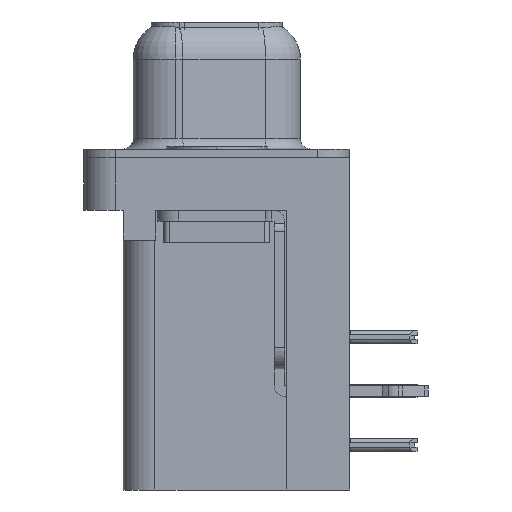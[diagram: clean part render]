
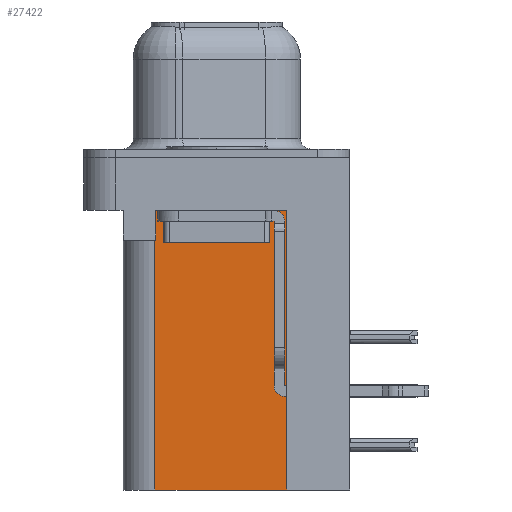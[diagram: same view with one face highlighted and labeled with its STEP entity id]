
A CAD part, left-side view. The second image highlights one B-rep face of the part: STEP entity #27422.
In plain terms, the highlighted planar face has unit normal (-1, 0, 0).
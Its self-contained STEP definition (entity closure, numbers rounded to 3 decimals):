
#402 = EDGE_CURVE ( 'NONE', #13520, #545, #34985, .T. ) ;
#545 = VERTEX_POINT ( 'NONE', #14239 ) ;
#626 = FACE_OUTER_BOUND ( 'NONE', #2961, .T. ) ;
#1063 = VECTOR ( 'NONE', #6918, 1000. ) ;
#1377 = DIRECTION ( 'NONE',  ( 0., 1., 0. ) ) ;
#2961 = EDGE_LOOP ( 'NONE', ( #30297, #29498, #32369, #11836, #6723, #16919 ) ) ;
#3932 = VERTEX_POINT ( 'NONE', #15063 ) ;
#4312 = CARTESIAN_POINT ( 'NONE',  ( 3.765, 2.925, -15.7 ) ) ;
#4485 = EDGE_CURVE ( 'NONE', #3932, #18294, #33084, .T. ) ;
#6150 = DIRECTION ( 'NONE',  ( 0., 0., -1. ) ) ;
#6723 = ORIENTED_EDGE ( 'NONE', *, *, #402, .F. ) ;
#6918 = DIRECTION ( 'NONE',  ( 0., 0., 1. ) ) ;
#7165 = CARTESIAN_POINT ( 'NONE',  ( 3.765, 2.925, -3.9 ) ) ;
#7405 = VECTOR ( 'NONE', #26990, 1000. ) ;
#7788 = DIRECTION ( 'NONE',  ( 0., 0., -1. ) ) ;
#7951 = CARTESIAN_POINT ( 'NONE',  ( 3.765, 2.895, -3.9 ) ) ;
#10080 = VECTOR ( 'NONE', #23283, 1000. ) ;
#11691 = VECTOR ( 'NONE', #28534, 1000. ) ;
#11836 = ORIENTED_EDGE ( 'NONE', *, *, #25884, .F. ) ;
#12033 = CARTESIAN_POINT ( 'NONE',  ( 3.765, -3.295, -15.7 ) ) ;
#13520 = VERTEX_POINT ( 'NONE', #12033 ) ;
#14239 = CARTESIAN_POINT ( 'NONE',  ( 3.765, 2.925, -15.7 ) ) ;
#14698 = LINE ( 'NONE', #23119, #1063 ) ;
#15063 = CARTESIAN_POINT ( 'NONE',  ( 3.765, 2.895, -2.5 ) ) ;
#16486 = VERTEX_POINT ( 'NONE', #18619 ) ;
#16892 = PLANE ( 'NONE',  #26796 ) ;
#16919 = ORIENTED_EDGE ( 'NONE', *, *, #24794, .T. ) ;
#17521 = CARTESIAN_POINT ( 'NONE',  ( 3.765, 2.895, -3.9 ) ) ;
#18294 = VERTEX_POINT ( 'NONE', #17521 ) ;
#18619 = CARTESIAN_POINT ( 'NONE',  ( 3.765, -3.295, -2.5 ) ) ;
#19478 = VECTOR ( 'NONE', #7788, 1000. ) ;
#19611 = CARTESIAN_POINT ( 'NONE',  ( 3.765, -3.295, -15.7 ) ) ;
#19941 = EDGE_CURVE ( 'NONE', #18294, #24805, #29804, .T. ) ;
#21555 = CARTESIAN_POINT ( 'NONE',  ( 3.765, 0., -3.9 ) ) ;
#22357 = DIRECTION ( 'NONE',  ( 1., 0., 0. ) ) ;
#23119 = CARTESIAN_POINT ( 'NONE',  ( 3.765, -3.295, -15.7 ) ) ;
#23283 = DIRECTION ( 'NONE',  ( 0., 0., 1. ) ) ;
#23562 = EDGE_CURVE ( 'NONE', #16486, #3932, #24557, .T. ) ;
#24557 = LINE ( 'NONE', #28454, #30896 ) ;
#24794 = EDGE_CURVE ( 'NONE', #13520, #16486, #14698, .T. ) ;
#24805 = VERTEX_POINT ( 'NONE', #7165 ) ;
#25884 = EDGE_CURVE ( 'NONE', #545, #24805, #30788, .T. ) ;
#26796 = AXIS2_PLACEMENT_3D ( 'NONE', #19611, #22357, #6150 ) ;
#26990 = DIRECTION ( 'NONE',  ( 0., 1., 0. ) ) ;
#27422 = ADVANCED_FACE ( 'NONE', ( #626 ), #16892, .F. ) ;
#28454 = CARTESIAN_POINT ( 'NONE',  ( 3.765, -3.295, -2.5 ) ) ;
#28509 = CARTESIAN_POINT ( 'NONE',  ( 3.765, -3.295, -15.7 ) ) ;
#28534 = DIRECTION ( 'NONE',  ( 0., 1., 0. ) ) ;
#29498 = ORIENTED_EDGE ( 'NONE', *, *, #4485, .T. ) ;
#29804 = LINE ( 'NONE', #21555, #7405 ) ;
#30297 = ORIENTED_EDGE ( 'NONE', *, *, #23562, .T. ) ;
#30788 = LINE ( 'NONE', #4312, #10080 ) ;
#30896 = VECTOR ( 'NONE', #1377, 1000. ) ;
#32369 = ORIENTED_EDGE ( 'NONE', *, *, #19941, .T. ) ;
#33084 = LINE ( 'NONE', #7951, #19478 ) ;
#34985 = LINE ( 'NONE', #28509, #11691 ) ;
